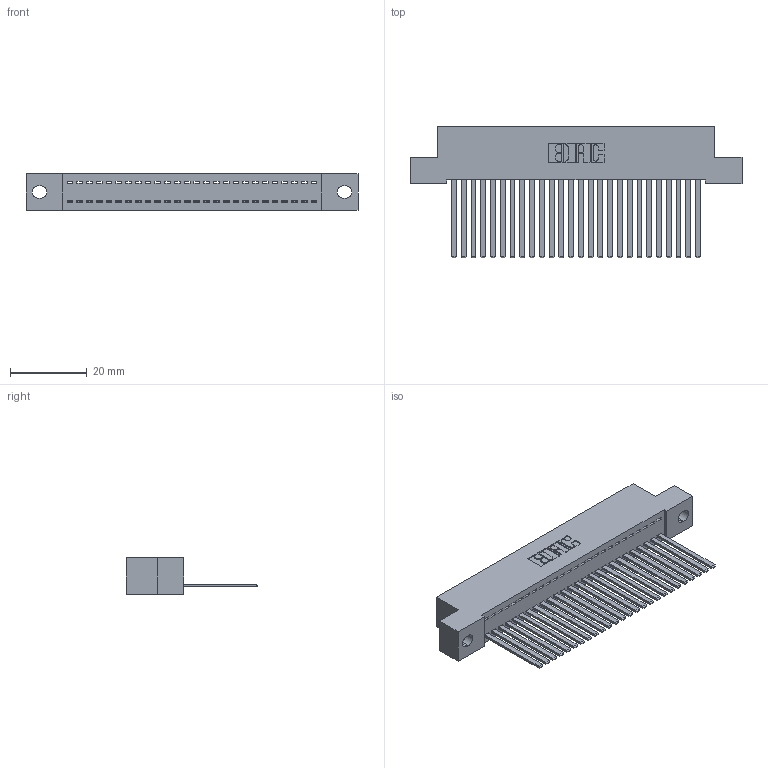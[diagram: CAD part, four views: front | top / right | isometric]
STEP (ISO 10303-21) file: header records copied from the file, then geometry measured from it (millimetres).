
FILE_DESCRIPTION (( 'STEP AP203' ), '1' );
FILE_NAME ('342-026-544-102.STEP', '2019-10-02T01:31:55', ( '' ), ( '' ), 'SwSTEP 2.0', 'SolidWorks 2016', '' );
FILE_SCHEMA (( 'CONFIG_CONTROL_DESIGN' ));
Length unit declared in the file: inch
Products named in the file (3): 342 Part_.128 Slot; 345-292-001_345-293-144; 342-026-544-102
Assembly tree (27 placements, depth 2):
  342-026-544-102
    342 Part_.128 Slot
    345-292-001_345-293-144  x26
Bounding box: 86.36 x 34.3 x 9.4 mm (x, y, z)
Volume: 7762.1 mm3; surface area: 11716.1 mm2
Topology: 27 solids, 27 shells, 1466 faces, 4419 edges, 2910 vertices
Faces by surface type: plane 1058, cylinder 408
Entity records: 17783 total; most frequent: CARTESIAN_POINT 3076, ORIENTED_EDGE 3038, DIRECTION 2623, EDGE_CURVE 1519, VECTOR 1395, LINE 1395, VERTEX_POINT 1010, AXIS2_PLACEMENT_3D 614
